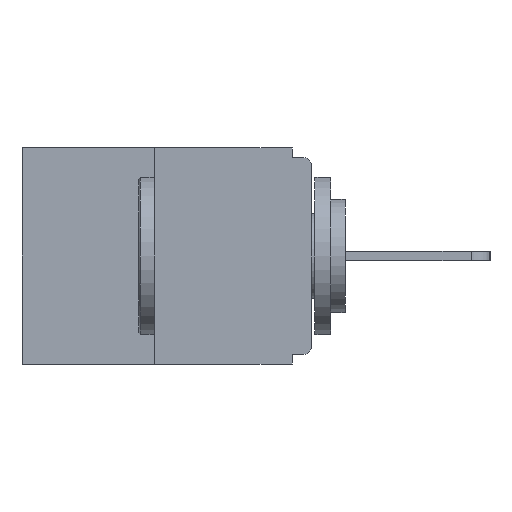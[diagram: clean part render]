
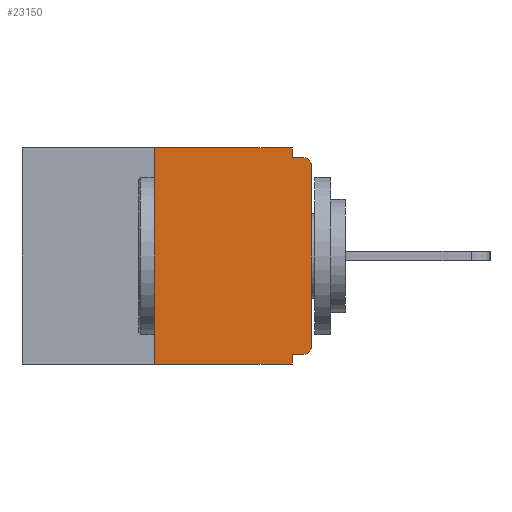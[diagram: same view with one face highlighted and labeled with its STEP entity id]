
A CAD part, left-side view. The second image highlights one B-rep face of the part: STEP entity #23150.
In plain terms, the highlighted planar face has unit normal (-1, 0, 0).
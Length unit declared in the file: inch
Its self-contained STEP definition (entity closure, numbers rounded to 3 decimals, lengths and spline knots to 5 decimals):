
#235 = VERTEX_POINT ( 'NONE', #6915 ) ;
#517 = CARTESIAN_POINT ( 'NONE',  ( 0., 0.015, -0.328 ) ) ;
#586 = EDGE_CURVE ( 'NONE', #9956, #235, #1403, .T. ) ;
#662 = EDGE_LOOP ( 'NONE', ( #19411, #22712, #17921, #12548, #6942, #18597, #2023, #21101, #2299, #11643 ) ) ;
#1062 = EDGE_CURVE ( 'NONE', #9509, #22826, #4565, .T. ) ;
#1140 = CARTESIAN_POINT ( 'NONE',  ( 0., 0., -0.328 ) ) ;
#1403 = LINE ( 'NONE', #1140, #9278 ) ;
#1535 = CARTESIAN_POINT ( 'NONE',  ( 0., 0.031, 0. ) ) ;
#1649 = VECTOR ( 'NONE', #2102, 39.37008 ) ;
#1809 = DIRECTION ( 'NONE',  ( -1., 0., 0. ) ) ;
#1868 = DIRECTION ( 'NONE',  ( -1., 0., 0. ) ) ;
#2023 = ORIENTED_EDGE ( 'NONE', *, *, #16881, .T. ) ;
#2064 = VERTEX_POINT ( 'NONE', #14562 ) ;
#2102 = DIRECTION ( 'NONE',  ( 0., 0., -1. ) ) ;
#2299 = ORIENTED_EDGE ( 'NONE', *, *, #15062, .F. ) ;
#2382 = VERTEX_POINT ( 'NONE', #12896 ) ;
#2444 = EDGE_CURVE ( 'NONE', #9956, #2382, #23064, .T. ) ;
#3217 = LINE ( 'NONE', #21834, #16602 ) ;
#3248 = LINE ( 'NONE', #15569, #23637 ) ;
#3462 = EDGE_CURVE ( 'NONE', #2064, #5174, #3217, .T. ) ;
#3507 = CARTESIAN_POINT ( 'NONE',  ( 0., 0.031, -0.015 ) ) ;
#3582 = PLANE ( 'NONE',  #17828 ) ;
#3666 = VECTOR ( 'NONE', #20939, 39.37008 ) ;
#4168 = EDGE_CURVE ( 'NONE', #5174, #24810, #22220, .T. ) ;
#4565 = LINE ( 'NONE', #18969, #3666 ) ;
#5174 = VERTEX_POINT ( 'NONE', #18654 ) ;
#5635 = CARTESIAN_POINT ( 'NONE',  ( 0., 0.25, 0. ) ) ;
#5766 = VERTEX_POINT ( 'NONE', #19640 ) ;
#6328 = DIRECTION ( 'NONE',  ( 0., -1., 0. ) ) ;
#6716 = CARTESIAN_POINT ( 'NONE',  ( 0., 0., -0.015 ) ) ;
#6915 = CARTESIAN_POINT ( 'NONE',  ( 0., 0.031, -0.328 ) ) ;
#6942 = ORIENTED_EDGE ( 'NONE', *, *, #586, .F. ) ;
#7354 = CIRCLE ( 'NONE', #20060, 0.015 ) ;
#7428 = LINE ( 'NONE', #6716, #22043 ) ;
#8233 = VERTEX_POINT ( 'NONE', #17811 ) ;
#9278 = VECTOR ( 'NONE', #18639, 39.37008 ) ;
#9283 = AXIS2_PLACEMENT_3D ( 'NONE', #19322, #1809, #13482 ) ;
#9431 = CARTESIAN_POINT ( 'NONE',  ( 0., 0.46, 0. ) ) ;
#9509 = VERTEX_POINT ( 'NONE', #14142 ) ;
#9531 = DIRECTION ( 'NONE',  ( 0., 0., 1. ) ) ;
#9956 = VERTEX_POINT ( 'NONE', #517 ) ;
#10291 = EDGE_CURVE ( 'NONE', #235, #22826, #14663, .T. ) ;
#11543 = CARTESIAN_POINT ( 'NONE',  ( 0., 0.015, -0.03 ) ) ;
#11643 = ORIENTED_EDGE ( 'NONE', *, *, #4168, .F. ) ;
#12337 = VECTOR ( 'NONE', #22580, 39.37008 ) ;
#12548 = ORIENTED_EDGE ( 'NONE', *, *, #10291, .F. ) ;
#12896 = CARTESIAN_POINT ( 'NONE',  ( 0., 0., -0.313 ) ) ;
#13338 = DIRECTION ( 'NONE',  ( 0., 0., -1. ) ) ;
#13369 = EDGE_CURVE ( 'NONE', #8233, #5766, #7354, .T. ) ;
#13482 = DIRECTION ( 'NONE',  ( 0., 0., -1. ) ) ;
#14142 = CARTESIAN_POINT ( 'NONE',  ( 0., 0.25, -0.343 ) ) ;
#14146 = VECTOR ( 'NONE', #9531, 39.37008 ) ;
#14562 = CARTESIAN_POINT ( 'NONE',  ( 0., 0.25, 0. ) ) ;
#14617 = DIRECTION ( 'NONE',  ( 0., -1., 0. ) ) ;
#14663 = LINE ( 'NONE', #17806, #1649 ) ;
#15062 = EDGE_CURVE ( 'NONE', #24810, #5766, #7428, .T. ) ;
#15569 = CARTESIAN_POINT ( 'NONE',  ( 0., 0., 0. ) ) ;
#16602 = VECTOR ( 'NONE', #6328, 39.37008 ) ;
#16881 = EDGE_CURVE ( 'NONE', #2382, #8233, #3248, .T. ) ;
#17179 = DIRECTION ( 'NONE',  ( 1., 0., 0. ) ) ;
#17806 = CARTESIAN_POINT ( 'NONE',  ( 0., 0.031, -0.343 ) ) ;
#17811 = CARTESIAN_POINT ( 'NONE',  ( 0., 0., -0.03 ) ) ;
#17828 = AXIS2_PLACEMENT_3D ( 'NONE', #9431, #17179, #13338 ) ;
#17921 = ORIENTED_EDGE ( 'NONE', *, *, #1062, .T. ) ;
#18442 = LINE ( 'NONE', #5635, #14146 ) ;
#18597 = ORIENTED_EDGE ( 'NONE', *, *, #2444, .T. ) ;
#18623 = FACE_OUTER_BOUND ( 'NONE', #662, .T. ) ;
#18639 = DIRECTION ( 'NONE',  ( 0., 1., 0. ) ) ;
#18654 = CARTESIAN_POINT ( 'NONE',  ( 0., 0.031, 0. ) ) ;
#18969 = CARTESIAN_POINT ( 'NONE',  ( 0., 0.46, -0.343 ) ) ;
#19322 = CARTESIAN_POINT ( 'NONE',  ( 0., 0.015, -0.313 ) ) ;
#19411 = ORIENTED_EDGE ( 'NONE', *, *, #3462, .F. ) ;
#19640 = CARTESIAN_POINT ( 'NONE',  ( 0., 0.015, -0.015 ) ) ;
#20060 = AXIS2_PLACEMENT_3D ( 'NONE', #11543, #1868, #23272 ) ;
#20939 = DIRECTION ( 'NONE',  ( 0., -1., 0. ) ) ;
#21101 = ORIENTED_EDGE ( 'NONE', *, *, #13369, .T. ) ;
#21105 = DIRECTION ( 'NONE',  ( 0., 0., 1. ) ) ;
#21834 = CARTESIAN_POINT ( 'NONE',  ( 0., 0.46, 0. ) ) ;
#22043 = VECTOR ( 'NONE', #14617, 39.37008 ) ;
#22220 = LINE ( 'NONE', #1535, #12337 ) ;
#22580 = DIRECTION ( 'NONE',  ( 0., 0., -1. ) ) ;
#22712 = ORIENTED_EDGE ( 'NONE', *, *, #24754, .F. ) ;
#22826 = VERTEX_POINT ( 'NONE', #24700 ) ;
#23064 = CIRCLE ( 'NONE', #9283, 0.015 ) ;
#23150 = ADVANCED_FACE ( 'NONE', ( #18623 ), #3582, .F. ) ;
#23272 = DIRECTION ( 'NONE',  ( 0., 0., -1. ) ) ;
#23637 = VECTOR ( 'NONE', #21105, 39.37008 ) ;
#24700 = CARTESIAN_POINT ( 'NONE',  ( 0., 0.031, -0.343 ) ) ;
#24754 = EDGE_CURVE ( 'NONE', #9509, #2064, #18442, .T. ) ;
#24810 = VERTEX_POINT ( 'NONE', #3507 ) ;
